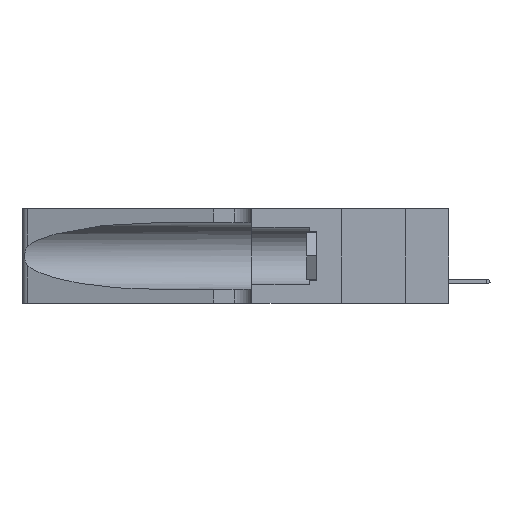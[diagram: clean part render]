
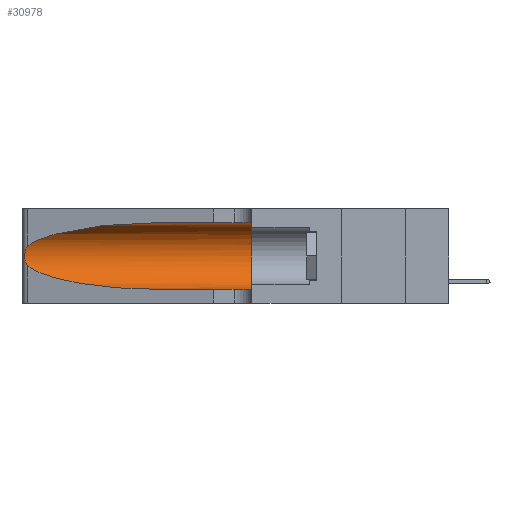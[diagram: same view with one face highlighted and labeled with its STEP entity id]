
A CAD part, left-side view. The second image highlights one B-rep face of the part: STEP entity #30978.
In plain terms, the highlighted cylindrical face has radius 3.308 mm (diameter 6.617 mm), a partial arc.
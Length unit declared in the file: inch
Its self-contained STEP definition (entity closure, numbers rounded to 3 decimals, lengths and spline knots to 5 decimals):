
#319 = CARTESIAN_POINT ( 'NONE',  ( 0.1305, 0.72297, 0.31525 ) ) ;
#1399 = EDGE_CURVE ( 'NONE', #25433, #12759, #16861, .T. ) ;
#1426 = CARTESIAN_POINT ( 'NONE',  ( 0.25856, 1.23593, 0.16098 ) ) ;
#1487 = DIRECTION ( 'NONE',  ( 0., 1., 0. ) ) ;
#2388 = CYLINDRICAL_SURFACE ( 'NONE', #27488, 0.13025 ) ;
#2837 = FACE_OUTER_BOUND ( 'NONE', #24383, .T. ) ;
#4093 = CARTESIAN_POINT ( 'NONE',  ( 0.25789, 1.23486, 0.15765 ) ) ;
#4190 = CIRCLE ( 'NONE', #31216, 0.13025 ) ;
#4220 = CARTESIAN_POINT ( 'NONE',  ( 0.25639, 1.23184, 0.21858 ) ) ;
#6040 =( BOUNDED_CURVE ( )  B_SPLINE_CURVE ( 3, ( #22867, #31775, #18210, #18073 ),
 .UNSPECIFIED., .F., .F. ) 
 B_SPLINE_CURVE_WITH_KNOTS ( ( 4, 4 ),
 ( 1.5708, 2.84003 ),
 .UNSPECIFIED. ) 
 CURVE ( )  GEOMETRIC_REPRESENTATION_ITEM ( )  RATIONAL_B_SPLINE_CURVE ( ( 1., 0.87, 0.87, 1. ) ) 
 REPRESENTATION_ITEM ( '' )  );
#6452 = ORIENTED_EDGE ( 'NONE', *, *, #34868, .T. ) ;
#8306 = CARTESIAN_POINT ( 'NONE',  ( 0.18966, 0.96281, 0.05475 ) ) ;
#9876 = VECTOR ( 'NONE', #24897, 39.37008 ) ;
#9892 = CARTESIAN_POINT ( 'NONE',  ( 0.26075, 1.23896, 0.19203 ) ) ;
#10121 = CARTESIAN_POINT ( 'NONE',  ( 0.1305, 0.35, 0.31525 ) ) ;
#10211 = DIRECTION ( 'NONE',  ( 0., 0., 1. ) ) ;
#10304 = CARTESIAN_POINT ( 'NONE',  ( 0.25487, 1.22718, 0.14631 ) ) ;
#12307 = DIRECTION ( 'NONE',  ( 0., -1., 0. ) ) ;
#12593 = CARTESIAN_POINT ( 'NONE',  ( 0.1305, 1.61858, 0.31525 ) ) ;
#12759 = VERTEX_POINT ( 'NONE', #10121 ) ;
#13141 = CARTESIAN_POINT ( 'NONE',  ( 0.25854, 1.2359, 0.20912 ) ) ;
#13269 = CARTESIAN_POINT ( 'NONE',  ( 0.25555, 1.22994, 0.2215 ) ) ;
#13868 = CARTESIAN_POINT ( 'NONE',  ( 0.25487, 1.22718, 0.14631 ) ) ;
#14095 = ORIENTED_EDGE ( 'NONE', *, *, #16689, .F. ) ;
#16689 = EDGE_CURVE ( 'NONE', #12759, #33933, #4190, .T. ) ;
#16861 = LINE ( 'NONE', #12593, #9876 ) ;
#17509 = CARTESIAN_POINT ( 'NONE',  ( 0.1305, 1.61858, 0.185 ) ) ;
#17522 = VERTEX_POINT ( 'NONE', #33383 ) ;
#18073 = CARTESIAN_POINT ( 'NONE',  ( 0.25487, 1.22718, 0.22369 ) ) ;
#18210 = CARTESIAN_POINT ( 'NONE',  ( 0.2373, 1.15595, 0.28018 ) ) ;
#18273 = LINE ( 'NONE', #27181, #27515 ) ;
#18845 = CARTESIAN_POINT ( 'NONE',  ( 0.26075, 1.23896, 0.178 ) ) ;
#19111 = CARTESIAN_POINT ( 'NONE',  ( 0.26018, 1.23835, 0.19895 ) ) ;
#19247 = CARTESIAN_POINT ( 'NONE',  ( 0.25487, 1.22718, 0.14631 ) ) ;
#19670 = EDGE_CURVE ( 'NONE', #37083, #33933, #18273, .T. ) ;
#20204 = CARTESIAN_POINT ( 'NONE',  ( 0.1305, 0.72297, 0.05475 ) ) ;
#21605 = ORIENTED_EDGE ( 'NONE', *, *, #28916, .T. ) ;
#22087 = CARTESIAN_POINT ( 'NONE',  ( 0.25639, 1.23186, 0.15144 ) ) ;
#22212 = CARTESIAN_POINT ( 'NONE',  ( 0.26017, 1.23833, 0.17102 ) ) ;
#22867 = CARTESIAN_POINT ( 'NONE',  ( 0.1305, 0.72297, 0.31525 ) ) ;
#23711 = CARTESIAN_POINT ( 'NONE',  ( 0.1305, 0.72297, 0.05475 ) ) ;
#24267 = CARTESIAN_POINT ( 'NONE',  ( 0.1305, 0.35, 0.05475 ) ) ;
#24383 = EDGE_LOOP ( 'NONE', ( #21605, #6452, #37986, #27946, #14095, #33370 ) ) ;
#24479 = B_SPLINE_CURVE_WITH_KNOTS ( 'NONE', 3,
 ( #27612, #13269, #4220, #30855, #13141, #19111, #9892, #18845, #22212, #1426, #4093, #22087, #25050, #19247 ),
 .UNSPECIFIED., .F., .F.,
 ( 4, 2, 2, 2, 2, 2, 4 ),
 ( 0., 0.00027, 0.00053, 0.00107, 0.0016, 0.00187, 0.00214 ),
 .UNSPECIFIED. ) ;
#24833 = CARTESIAN_POINT ( 'NONE',  ( 0.1305, 0.35, 0.185 ) ) ;
#24897 = DIRECTION ( 'NONE',  ( 0., -1., 0. ) ) ;
#25050 = CARTESIAN_POINT ( 'NONE',  ( 0.25555, 1.22993, 0.14849 ) ) ;
#25433 = VERTEX_POINT ( 'NONE', #319 ) ;
#26560 = DIRECTION ( 'NONE',  ( 0., -1., 0. ) ) ;
#26852 = VERTEX_POINT ( 'NONE', #10304 ) ;
#27181 = CARTESIAN_POINT ( 'NONE',  ( 0.1305, 1.61858, 0.05475 ) ) ;
#27488 = AXIS2_PLACEMENT_3D ( 'NONE', #17509, #26560, #29639 ) ;
#27515 = VECTOR ( 'NONE', #12307, 39.37008 ) ;
#27612 = CARTESIAN_POINT ( 'NONE',  ( 0.25487, 1.22718, 0.22369 ) ) ;
#27946 = ORIENTED_EDGE ( 'NONE', *, *, #19670, .T. ) ;
#28916 = EDGE_CURVE ( 'NONE', #25433, #17522, #6040, .T. ) ;
#29639 = DIRECTION ( 'NONE',  ( 0., 0., -1. ) ) ;
#30855 = CARTESIAN_POINT ( 'NONE',  ( 0.25787, 1.23484, 0.2124 ) ) ;
#30978 = ADVANCED_FACE ( 'NONE', ( #2837 ), #2388, .F. ) ;
#31216 = AXIS2_PLACEMENT_3D ( 'NONE', #24833, #1487, #10211 ) ;
#31775 = CARTESIAN_POINT ( 'NONE',  ( 0.18966, 0.96281, 0.31525 ) ) ;
#31839 = CARTESIAN_POINT ( 'NONE',  ( 0.2373, 1.15595, 0.08982 ) ) ;
#33370 = ORIENTED_EDGE ( 'NONE', *, *, #1399, .F. ) ;
#33383 = CARTESIAN_POINT ( 'NONE',  ( 0.25487, 1.22718, 0.22369 ) ) ;
#33933 = VERTEX_POINT ( 'NONE', #24267 ) ;
#34868 = EDGE_CURVE ( 'NONE', #17522, #26852, #24479, .T. ) ;
#37083 = VERTEX_POINT ( 'NONE', #23711 ) ;
#37610 =( BOUNDED_CURVE ( )  B_SPLINE_CURVE ( 3, ( #13868, #31839, #8306, #20204 ),
 .UNSPECIFIED., .F., .F. ) 
 B_SPLINE_CURVE_WITH_KNOTS ( ( 4, 4 ),
 ( 3.44316, 4.71239 ),
 .UNSPECIFIED. ) 
 CURVE ( )  GEOMETRIC_REPRESENTATION_ITEM ( )  RATIONAL_B_SPLINE_CURVE ( ( 1., 0.87, 0.87, 1. ) ) 
 REPRESENTATION_ITEM ( '' )  );
#37986 = ORIENTED_EDGE ( 'NONE', *, *, #38313, .T. ) ;
#38313 = EDGE_CURVE ( 'NONE', #26852, #37083, #37610, .T. ) ;
